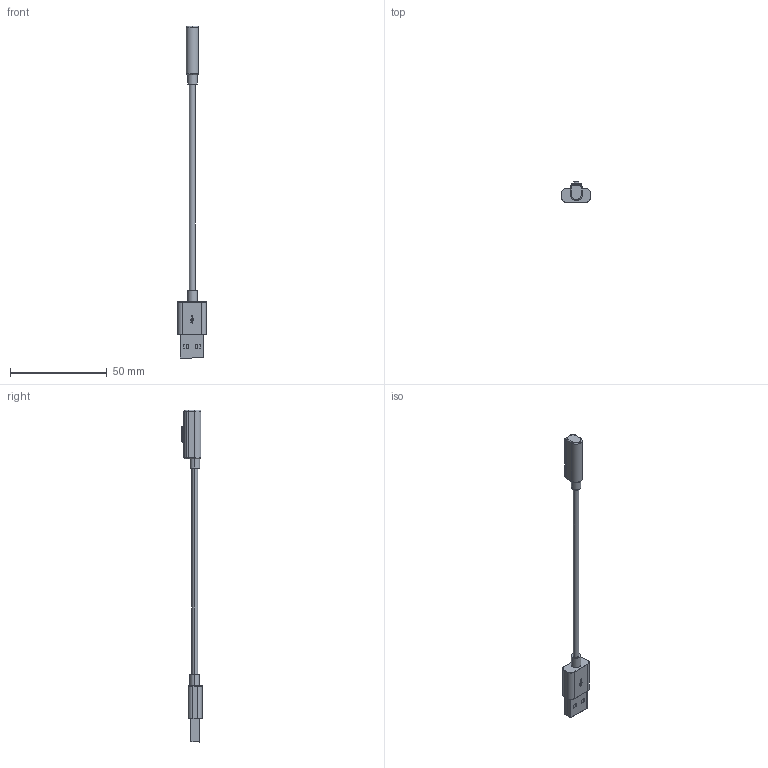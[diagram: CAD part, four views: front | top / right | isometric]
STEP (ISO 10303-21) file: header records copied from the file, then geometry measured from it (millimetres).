
FILE_DESCRIPTION (( 'STEP AP214' ), '1' );
FILE_NAME ('687L0421A501200.STEP', '2023-05-16T12:57:56', ( '' ), ( '' ), 'SwSTEP 2.0', 'SolidWorks 2020', '' );
FILE_SCHEMA (( 'AUTOMOTIVE_DESIGN' ));
Length unit declared in the file: millimetre
Products named in the file (1): 687L0421A501200
Bounding box: 15 x 10.45 x 171.98 mm (x, y, z)
Volume: 4292.6 mm3; surface area: 3910 mm2
Topology: 7 solids, 9 shells, 291 faces, 687 edges, 434 vertices
Faces by surface type: plane 156, cylinder 83, cone 20, torus 18, bspline 14
Entity records: 12099 total; most frequent: CARTESIAN_POINT 2333, DIRECTION 1365, ORIENTED_EDGE 1358, EDGE_CURVE 679, AXIS2_PLACEMENT_3D 464, VECTOR 437, LINE 437, VERTEX_POINT 434
